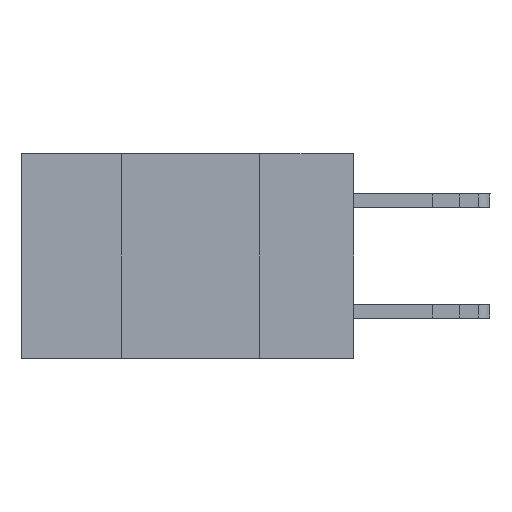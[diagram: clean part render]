
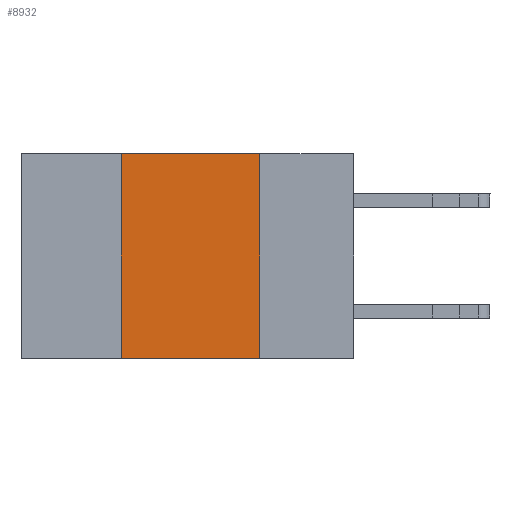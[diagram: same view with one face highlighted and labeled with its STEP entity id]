
A CAD part, left-side view. The second image highlights one B-rep face of the part: STEP entity #8932.
In plain terms, the highlighted planar face has unit normal (-1, 0, 0).
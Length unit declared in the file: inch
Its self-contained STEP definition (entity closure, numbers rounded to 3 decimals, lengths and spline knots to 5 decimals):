
#66 = DIRECTION ( 'NONE',  ( 0., 0., -1. ) ) ;
#2603 = CARTESIAN_POINT ( 'NONE',  ( 0., 0.6, 0. ) ) ;
#2841 = VERTEX_POINT ( 'NONE', #3957 ) ;
#3417 = DIRECTION ( 'NONE',  ( 0., -1., 0. ) ) ;
#3926 = CARTESIAN_POINT ( 'NONE',  ( 0., 0.17, -0.37 ) ) ;
#3957 = CARTESIAN_POINT ( 'NONE',  ( 0., 0.42, 0. ) ) ;
#4152 = VERTEX_POINT ( 'NONE', #11186 ) ;
#5460 = LINE ( 'NONE', #20191, #7000 ) ;
#5509 = ORIENTED_EDGE ( 'NONE', *, *, #18464, .F. ) ;
#6140 = EDGE_CURVE ( 'NONE', #4152, #2841, #5460, .T. ) ;
#6644 = ORIENTED_EDGE ( 'NONE', *, *, #11060, .T. ) ;
#6681 = CARTESIAN_POINT ( 'NONE',  ( 0., 0.6, -0.37 ) ) ;
#7000 = VECTOR ( 'NONE', #18308, 39.37008 ) ;
#8436 = VECTOR ( 'NONE', #13114, 39.37008 ) ;
#8932 = ADVANCED_FACE ( 'NONE', ( #10724 ), #15599, .F. ) ;
#9099 = LINE ( 'NONE', #6681, #8436 ) ;
#10587 = DIRECTION ( 'NONE',  ( 0., 0., -1. ) ) ;
#10724 = FACE_OUTER_BOUND ( 'NONE', #20761, .T. ) ;
#11060 = EDGE_CURVE ( 'NONE', #4152, #18011, #9099, .T. ) ;
#11186 = CARTESIAN_POINT ( 'NONE',  ( 0., 0.42, -0.37 ) ) ;
#11293 = DIRECTION ( 'NONE',  ( 1., 0., 0. ) ) ;
#11455 = LINE ( 'NONE', #20194, #14032 ) ;
#11955 = VERTEX_POINT ( 'NONE', #25566 ) ;
#13114 = DIRECTION ( 'NONE',  ( 0., -1., 0. ) ) ;
#14032 = VECTOR ( 'NONE', #3417, 39.37008 ) ;
#14911 = ORIENTED_EDGE ( 'NONE', *, *, #6140, .F. ) ;
#15599 = PLANE ( 'NONE',  #24457 ) ;
#16038 = EDGE_CURVE ( 'NONE', #2841, #11955, #11455, .T. ) ;
#18011 = VERTEX_POINT ( 'NONE', #3926 ) ;
#18308 = DIRECTION ( 'NONE',  ( 0., 0., 1. ) ) ;
#18464 = EDGE_CURVE ( 'NONE', #11955, #18011, #27805, .T. ) ;
#20191 = CARTESIAN_POINT ( 'NONE',  ( 0., 0.42, 0. ) ) ;
#20194 = CARTESIAN_POINT ( 'NONE',  ( 0., 0.6, 0. ) ) ;
#20761 = EDGE_LOOP ( 'NONE', ( #5509, #26182, #14911, #6644 ) ) ;
#23042 = CARTESIAN_POINT ( 'NONE',  ( 0., 0.17, 0. ) ) ;
#24457 = AXIS2_PLACEMENT_3D ( 'NONE', #2603, #11293, #66 ) ;
#25566 = CARTESIAN_POINT ( 'NONE',  ( 0., 0.17, 0. ) ) ;
#25568 = VECTOR ( 'NONE', #10587, 39.37008 ) ;
#26182 = ORIENTED_EDGE ( 'NONE', *, *, #16038, .F. ) ;
#27805 = LINE ( 'NONE', #23042, #25568 ) ;
